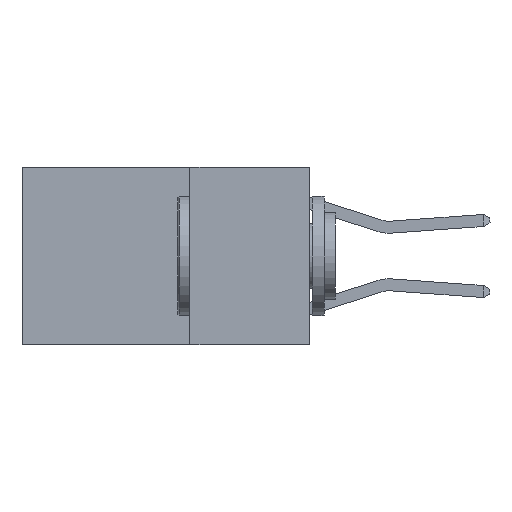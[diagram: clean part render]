
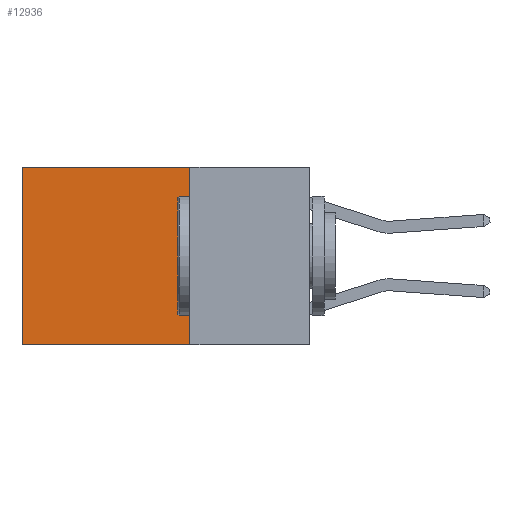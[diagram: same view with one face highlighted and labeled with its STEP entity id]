
A CAD part, left-side view. The second image highlights one B-rep face of the part: STEP entity #12936.
In plain terms, the highlighted planar face has unit normal (-1, 0, 0).
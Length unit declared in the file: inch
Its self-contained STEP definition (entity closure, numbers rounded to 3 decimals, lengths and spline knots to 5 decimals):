
#99 = CARTESIAN_POINT ( 'NONE',  ( 0.2625, 0.25, -0.37 ) ) ;
#415 = LINE ( 'NONE', #5711, #7985 ) ;
#1092 = EDGE_CURVE ( 'NONE', #4150, #3234, #415, .T. ) ;
#1432 = DIRECTION ( 'NONE',  ( 0., 1., 0. ) ) ;
#3234 = VERTEX_POINT ( 'NONE', #14268 ) ;
#4051 = DIRECTION ( 'NONE',  ( 0., 0., -1. ) ) ;
#4150 = VERTEX_POINT ( 'NONE', #9983 ) ;
#4197 = AXIS2_PLACEMENT_3D ( 'NONE', #6106, #11664, #7710 ) ;
#4245 = CARTESIAN_POINT ( 'NONE',  ( 0.2625, 0.25, 0. ) ) ;
#4425 = LINE ( 'NONE', #12363, #8531 ) ;
#5276 = VECTOR ( 'NONE', #1432, 39.37008 ) ;
#5711 = CARTESIAN_POINT ( 'NONE',  ( 0.2625, 0.6, 0. ) ) ;
#6106 = CARTESIAN_POINT ( 'NONE',  ( 0.2625, 0.25, 0. ) ) ;
#6886 = DIRECTION ( 'NONE',  ( 0., 1., 0. ) ) ;
#7150 = DIRECTION ( 'NONE',  ( 0., 0., -1. ) ) ;
#7251 = VECTOR ( 'NONE', #4051, 39.37008 ) ;
#7710 = DIRECTION ( 'NONE',  ( 0., 0., -1. ) ) ;
#7985 = VECTOR ( 'NONE', #7150, 39.37008 ) ;
#8015 = VERTEX_POINT ( 'NONE', #16441 ) ;
#8531 = VECTOR ( 'NONE', #6886, 39.37008 ) ;
#8716 = ORIENTED_EDGE ( 'NONE', *, *, #11537, .F. ) ;
#8921 = EDGE_CURVE ( 'NONE', #15943, #4150, #4425, .T. ) ;
#9150 = LINE ( 'NONE', #99, #5276 ) ;
#9983 = CARTESIAN_POINT ( 'NONE',  ( 0.2625, 0.6, 0. ) ) ;
#10136 = EDGE_CURVE ( 'NONE', #15943, #8015, #13415, .T. ) ;
#11051 = FACE_OUTER_BOUND ( 'NONE', #14932, .T. ) ;
#11537 = EDGE_CURVE ( 'NONE', #8015, #3234, #9150, .T. ) ;
#11664 = DIRECTION ( 'NONE',  ( 1., 0., 0. ) ) ;
#11672 = ORIENTED_EDGE ( 'NONE', *, *, #8921, .T. ) ;
#12363 = CARTESIAN_POINT ( 'NONE',  ( 0.2625, 0.25, 0. ) ) ;
#12936 = ADVANCED_FACE ( 'NONE', ( #11051 ), #17295, .F. ) ;
#13415 = LINE ( 'NONE', #4245, #7251 ) ;
#13953 = CARTESIAN_POINT ( 'NONE',  ( 0.2625, 0.25, 0. ) ) ;
#14193 = ORIENTED_EDGE ( 'NONE', *, *, #10136, .F. ) ;
#14268 = CARTESIAN_POINT ( 'NONE',  ( 0.2625, 0.6, -0.37 ) ) ;
#14932 = EDGE_LOOP ( 'NONE', ( #17011, #8716, #14193, #11672 ) ) ;
#15943 = VERTEX_POINT ( 'NONE', #13953 ) ;
#16441 = CARTESIAN_POINT ( 'NONE',  ( 0.2625, 0.25, -0.37 ) ) ;
#17011 = ORIENTED_EDGE ( 'NONE', *, *, #1092, .T. ) ;
#17295 = PLANE ( 'NONE',  #4197 ) ;
